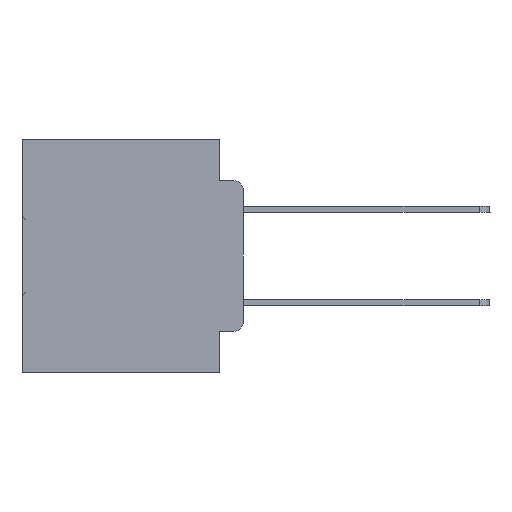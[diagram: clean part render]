
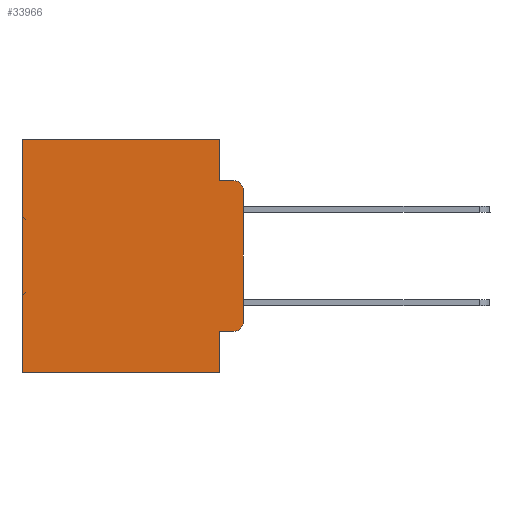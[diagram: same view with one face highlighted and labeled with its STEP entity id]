
A CAD part, left-side view. The second image highlights one B-rep face of the part: STEP entity #33966.
In plain terms, the highlighted planar face has unit normal (-1, 0, 0).
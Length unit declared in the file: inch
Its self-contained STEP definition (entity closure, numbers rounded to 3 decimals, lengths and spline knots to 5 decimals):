
#343 = VECTOR ( 'NONE', #28010, 39.37008 ) ;
#668 = VERTEX_POINT ( 'NONE', #3259 ) ;
#815 = LINE ( 'NONE', #27430, #33057 ) ;
#1588 = DIRECTION ( 'NONE',  ( 0., 1., 0. ) ) ;
#1662 = VECTOR ( 'NONE', #16810, 39.37008 ) ;
#3257 = ORIENTED_EDGE ( 'NONE', *, *, #12353, .F. ) ;
#3259 = CARTESIAN_POINT ( 'NONE',  ( 0.298, 0., -0.3915 ) ) ;
#3746 = DIRECTION ( 'NONE',  ( 0., 0., -1. ) ) ;
#4428 = VERTEX_POINT ( 'NONE', #27600 ) ;
#4653 = CARTESIAN_POINT ( 'NONE',  ( 0.298, 0.051, -0.0885 ) ) ;
#5111 = CARTESIAN_POINT ( 'NONE',  ( 0.298, 0., -0.1085 ) ) ;
#5295 = CIRCLE ( 'NONE', #8662, 0.02 ) ;
#5365 = ORIENTED_EDGE ( 'NONE', *, *, #26590, .T. ) ;
#6049 = ORIENTED_EDGE ( 'NONE', *, *, #20675, .F. ) ;
#6577 = CARTESIAN_POINT ( 'NONE',  ( 0.298, 0.473, 0. ) ) ;
#8053 = VECTOR ( 'NONE', #24718, 39.37008 ) ;
#8243 = VECTOR ( 'NONE', #23468, 39.37008 ) ;
#8472 = DIRECTION ( 'NONE',  ( 0., 0., -1. ) ) ;
#8662 = AXIS2_PLACEMENT_3D ( 'NONE', #24123, #35570, #26824 ) ;
#8714 = AXIS2_PLACEMENT_3D ( 'NONE', #35646, #24205, #27178 ) ;
#8814 = ORIENTED_EDGE ( 'NONE', *, *, #36915, .T. ) ;
#9135 = CARTESIAN_POINT ( 'NONE',  ( 0.298, 0.051, -0.5 ) ) ;
#10304 = FACE_OUTER_BOUND ( 'NONE', #16991, .T. ) ;
#11134 = DIRECTION ( 'NONE',  ( 1., 0., 0. ) ) ;
#11705 = CARTESIAN_POINT ( 'NONE',  ( 0.298, 0.02, -0.4115 ) ) ;
#11800 = LINE ( 'NONE', #18194, #8243 ) ;
#11961 = LINE ( 'NONE', #25331, #16031 ) ;
#12145 = VERTEX_POINT ( 'NONE', #15834 ) ;
#12353 = EDGE_CURVE ( 'NONE', #17529, #30333, #26377, .T. ) ;
#12487 = DIRECTION ( 'NONE',  ( 0., -1., 0. ) ) ;
#13086 = CARTESIAN_POINT ( 'NONE',  ( 0.298, 0., -0.5 ) ) ;
#13745 = EDGE_CURVE ( 'NONE', #28937, #668, #35302, .T. ) ;
#14185 = EDGE_CURVE ( 'NONE', #28937, #4428, #5295, .T. ) ;
#15834 = CARTESIAN_POINT ( 'NONE',  ( 0.298, 0.051, -0.4115 ) ) ;
#16031 = VECTOR ( 'NONE', #19187, 39.37008 ) ;
#16551 = EDGE_CURVE ( 'NONE', #27062, #668, #18991, .T. ) ;
#16555 = ORIENTED_EDGE ( 'NONE', *, *, #14185, .T. ) ;
#16810 = DIRECTION ( 'NONE',  ( 0., -1., 0. ) ) ;
#16991 = EDGE_LOOP ( 'NONE', ( #25942, #16555, #6049, #26756, #23773, #8814, #3257, #18437, #5365, #24854 ) ) ;
#17529 = VERTEX_POINT ( 'NONE', #9135 ) ;
#17825 = VERTEX_POINT ( 'NONE', #4653 ) ;
#18194 = CARTESIAN_POINT ( 'NONE',  ( 0.298, 0.051, 0. ) ) ;
#18437 = ORIENTED_EDGE ( 'NONE', *, *, #23231, .F. ) ;
#18991 = CIRCLE ( 'NONE', #8714, 0.02 ) ;
#19182 = LINE ( 'NONE', #21000, #30372 ) ;
#19187 = DIRECTION ( 'NONE',  ( 0., 0., -1. ) ) ;
#20338 = CARTESIAN_POINT ( 'NONE',  ( 0.298, 0.473, 0. ) ) ;
#20675 = EDGE_CURVE ( 'NONE', #17825, #4428, #30819, .T. ) ;
#21000 = CARTESIAN_POINT ( 'NONE',  ( 0.298, 0.051, -0.4115 ) ) ;
#23231 = EDGE_CURVE ( 'NONE', #12145, #17529, #11800, .T. ) ;
#23468 = DIRECTION ( 'NONE',  ( 0., 0., -1. ) ) ;
#23773 = ORIENTED_EDGE ( 'NONE', *, *, #25275, .T. ) ;
#24123 = CARTESIAN_POINT ( 'NONE',  ( 0.298, 0.02, -0.1085 ) ) ;
#24205 = DIRECTION ( 'NONE',  ( -1., 0., 0. ) ) ;
#24718 = DIRECTION ( 'NONE',  ( 0., 1., 0. ) ) ;
#24854 = ORIENTED_EDGE ( 'NONE', *, *, #16551, .T. ) ;
#25234 = VECTOR ( 'NONE', #8472, 39.37008 ) ;
#25275 = EDGE_CURVE ( 'NONE', #31756, #31140, #815, .T. ) ;
#25331 = CARTESIAN_POINT ( 'NONE',  ( 0.298, 0.051, 0. ) ) ;
#25942 = ORIENTED_EDGE ( 'NONE', *, *, #13745, .F. ) ;
#26210 = EDGE_CURVE ( 'NONE', #31756, #17825, #11961, .T. ) ;
#26377 = LINE ( 'NONE', #13086, #8053 ) ;
#26590 = EDGE_CURVE ( 'NONE', #12145, #27062, #19182, .T. ) ;
#26756 = ORIENTED_EDGE ( 'NONE', *, *, #26210, .F. ) ;
#26824 = DIRECTION ( 'NONE',  ( 0., 0., -1. ) ) ;
#27062 = VERTEX_POINT ( 'NONE', #11705 ) ;
#27178 = DIRECTION ( 'NONE',  ( 0., 0., -1. ) ) ;
#27430 = CARTESIAN_POINT ( 'NONE',  ( 0.298, 0., 0. ) ) ;
#27600 = CARTESIAN_POINT ( 'NONE',  ( 0.298, 0.02, -0.0885 ) ) ;
#28010 = DIRECTION ( 'NONE',  ( 0., 0., -1. ) ) ;
#28300 = PLANE ( 'NONE',  #34241 ) ;
#28937 = VERTEX_POINT ( 'NONE', #5111 ) ;
#30333 = VERTEX_POINT ( 'NONE', #34851 ) ;
#30372 = VECTOR ( 'NONE', #12487, 39.37008 ) ;
#30819 = LINE ( 'NONE', #31045, #1662 ) ;
#31045 = CARTESIAN_POINT ( 'NONE',  ( 0.298, 0.051, -0.0885 ) ) ;
#31140 = VERTEX_POINT ( 'NONE', #6577 ) ;
#31756 = VERTEX_POINT ( 'NONE', #32870 ) ;
#32578 = CARTESIAN_POINT ( 'NONE',  ( 0.298, 0., 0. ) ) ;
#32774 = LINE ( 'NONE', #20338, #25234 ) ;
#32870 = CARTESIAN_POINT ( 'NONE',  ( 0.298, 0.051, 0. ) ) ;
#33057 = VECTOR ( 'NONE', #1588, 39.37008 ) ;
#33966 = ADVANCED_FACE ( 'NONE', ( #10304 ), #28300, .F. ) ;
#34241 = AXIS2_PLACEMENT_3D ( 'NONE', #36770, #11134, #3746 ) ;
#34851 = CARTESIAN_POINT ( 'NONE',  ( 0.298, 0.473, -0.5 ) ) ;
#35302 = LINE ( 'NONE', #32578, #343 ) ;
#35570 = DIRECTION ( 'NONE',  ( -1., 0., 0. ) ) ;
#35646 = CARTESIAN_POINT ( 'NONE',  ( 0.298, 0.02, -0.3915 ) ) ;
#36770 = CARTESIAN_POINT ( 'NONE',  ( 0.298, 0., 0. ) ) ;
#36915 = EDGE_CURVE ( 'NONE', #31140, #30333, #32774, .T. ) ;
